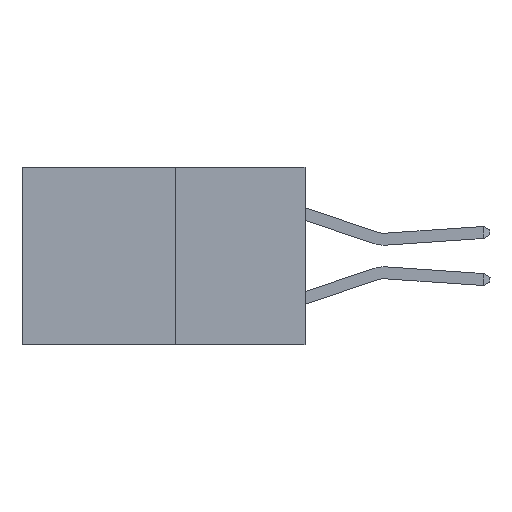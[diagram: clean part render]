
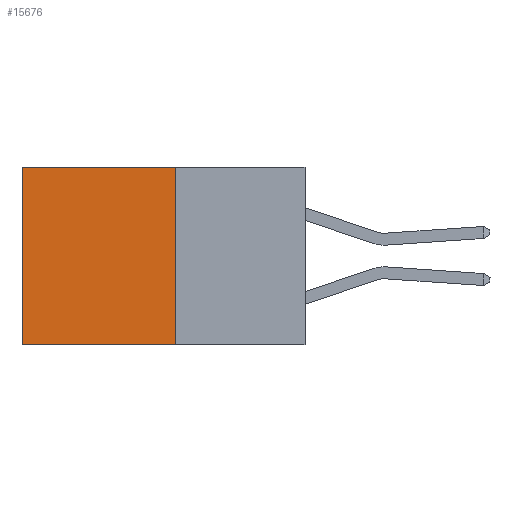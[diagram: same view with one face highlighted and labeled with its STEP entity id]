
A CAD part, left-side view. The second image highlights one B-rep face of the part: STEP entity #15676.
In plain terms, the highlighted planar face has unit normal (-1, 0, 0).
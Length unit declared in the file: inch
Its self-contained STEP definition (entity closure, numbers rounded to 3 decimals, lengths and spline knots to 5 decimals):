
#1017 = CARTESIAN_POINT ( 'NONE',  ( 0.277, 0.27, -0.37 ) ) ;
#2111 = VERTEX_POINT ( 'NONE', #3662 ) ;
#3662 = CARTESIAN_POINT ( 'NONE',  ( 0.277, 0.27, 0. ) ) ;
#3999 = EDGE_LOOP ( 'NONE', ( #12179, #13058, #15730, #26984 ) ) ;
#5647 = CARTESIAN_POINT ( 'NONE',  ( 0.277, 0.27, -0.37 ) ) ;
#5772 = EDGE_CURVE ( 'NONE', #12769, #26927, #10127, .T. ) ;
#7921 = LINE ( 'NONE', #30526, #13662 ) ;
#9329 = EDGE_CURVE ( 'NONE', #2111, #12769, #25847, .T. ) ;
#9449 = CARTESIAN_POINT ( 'NONE',  ( 0.277, 0.59, 0. ) ) ;
#10127 = LINE ( 'NONE', #1017, #15100 ) ;
#10571 = PLANE ( 'NONE',  #24915 ) ;
#11598 = VECTOR ( 'NONE', #25846, 39.37008 ) ;
#11784 = DIRECTION ( 'NONE',  ( 0., 0., -1. ) ) ;
#12179 = ORIENTED_EDGE ( 'NONE', *, *, #28383, .T. ) ;
#12352 = LINE ( 'NONE', #23409, #11598 ) ;
#12707 = FACE_OUTER_BOUND ( 'NONE', #3999, .T. ) ;
#12769 = VERTEX_POINT ( 'NONE', #16632 ) ;
#13007 = CARTESIAN_POINT ( 'NONE',  ( 0.277, 0.59, -0.37 ) ) ;
#13058 = ORIENTED_EDGE ( 'NONE', *, *, #5772, .F. ) ;
#13662 = VECTOR ( 'NONE', #23437, 39.37008 ) ;
#15100 = VECTOR ( 'NONE', #24232, 39.37008 ) ;
#15483 = DIRECTION ( 'NONE',  ( 0., 0., -1. ) ) ;
#15676 = ADVANCED_FACE ( 'NONE', ( #12707 ), #10571, .F. ) ;
#15730 = ORIENTED_EDGE ( 'NONE', *, *, #9329, .F. ) ;
#16632 = CARTESIAN_POINT ( 'NONE',  ( 0.277, 0.27, -0.37 ) ) ;
#23273 = EDGE_CURVE ( 'NONE', #2111, #31587, #12352, .T. ) ;
#23409 = CARTESIAN_POINT ( 'NONE',  ( 0.277, 0.27, 0. ) ) ;
#23437 = DIRECTION ( 'NONE',  ( 0., 0., -1. ) ) ;
#24232 = DIRECTION ( 'NONE',  ( 0., 1., 0. ) ) ;
#24311 = VECTOR ( 'NONE', #11784, 39.37008 ) ;
#24915 = AXIS2_PLACEMENT_3D ( 'NONE', #5647, #30069, #15483 ) ;
#25846 = DIRECTION ( 'NONE',  ( 0., 1., 0. ) ) ;
#25847 = LINE ( 'NONE', #26405, #24311 ) ;
#26405 = CARTESIAN_POINT ( 'NONE',  ( 0.277, 0.27, -0.37 ) ) ;
#26927 = VERTEX_POINT ( 'NONE', #13007 ) ;
#26984 = ORIENTED_EDGE ( 'NONE', *, *, #23273, .T. ) ;
#28383 = EDGE_CURVE ( 'NONE', #31587, #26927, #7921, .T. ) ;
#30069 = DIRECTION ( 'NONE',  ( 1., 0., 0. ) ) ;
#30526 = CARTESIAN_POINT ( 'NONE',  ( 0.277, 0.59, -0.37 ) ) ;
#31587 = VERTEX_POINT ( 'NONE', #9449 ) ;
